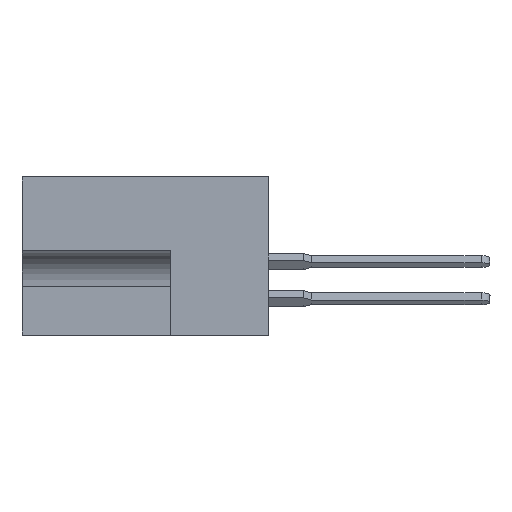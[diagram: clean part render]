
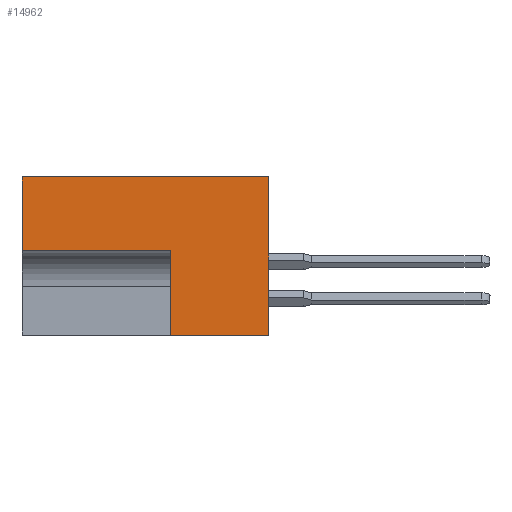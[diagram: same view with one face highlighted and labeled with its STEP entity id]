
A CAD part, left-side view. The second image highlights one B-rep face of the part: STEP entity #14962.
In plain terms, the highlighted planar face has unit normal (-1, 0, 0).
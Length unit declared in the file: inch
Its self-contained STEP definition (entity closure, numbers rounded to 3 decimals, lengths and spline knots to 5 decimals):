
#10 = DIRECTION ( 'NONE',  ( 0., 0., 1. ) ) ;
#1063 = LINE ( 'NONE', #12651, #9560 ) ;
#1127 = CARTESIAN_POINT ( 'NONE',  ( 0., 0.328, -0.248 ) ) ;
#2251 = DIRECTION ( 'NONE',  ( 0., -1., 0. ) ) ;
#2366 = VERTEX_POINT ( 'NONE', #2462 ) ;
#2462 = CARTESIAN_POINT ( 'NONE',  ( 0., 0., 0. ) ) ;
#3559 = DIRECTION ( 'NONE',  ( 0., 0., 1. ) ) ;
#3763 = ORIENTED_EDGE ( 'NONE', *, *, #11662, .F. ) ;
#5465 = VECTOR ( 'NONE', #10, 39.37008 ) ;
#5806 = ORIENTED_EDGE ( 'NONE', *, *, #26258, .T. ) ;
#5829 = VECTOR ( 'NONE', #8602, 39.37008 ) ;
#6051 = CARTESIAN_POINT ( 'NONE',  ( 0., 0.453, 0. ) ) ;
#6101 = ORIENTED_EDGE ( 'NONE', *, *, #23024, .T. ) ;
#6243 = VERTEX_POINT ( 'NONE', #10524 ) ;
#7580 = CARTESIAN_POINT ( 'NONE',  ( 0., 0.328, -0.531 ) ) ;
#8602 = DIRECTION ( 'NONE',  ( 0., 0., 1. ) ) ;
#9388 = EDGE_CURVE ( 'NONE', #23290, #2366, #15362, .T. ) ;
#9560 = VECTOR ( 'NONE', #2251, 39.37008 ) ;
#10290 = CARTESIAN_POINT ( 'NONE',  ( 0., 0., 0. ) ) ;
#10362 = LINE ( 'NONE', #10290, #5465 ) ;
#10475 = VECTOR ( 'NONE', #19140, 39.37008 ) ;
#10524 = CARTESIAN_POINT ( 'NONE',  ( 0., 0.328, -0.531 ) ) ;
#10763 = ORIENTED_EDGE ( 'NONE', *, *, #9388, .F. ) ;
#10971 = VERTEX_POINT ( 'NONE', #1127 ) ;
#11045 = LINE ( 'NONE', #16921, #5829 ) ;
#11230 = EDGE_CURVE ( 'NONE', #14862, #23290, #11045, .T. ) ;
#11662 = EDGE_CURVE ( 'NONE', #6243, #10971, #18782, .T. ) ;
#12002 = VECTOR ( 'NONE', #3559, 39.37008 ) ;
#12344 = DIRECTION ( 'NONE',  ( 0., -1., 0. ) ) ;
#12651 = CARTESIAN_POINT ( 'NONE',  ( 0., 0.453, -0.531 ) ) ;
#13093 = CARTESIAN_POINT ( 'NONE',  ( 0., 0.328, -0.248 ) ) ;
#13828 = PLANE ( 'NONE',  #17831 ) ;
#14303 = EDGE_LOOP ( 'NONE', ( #17032, #26651, #3763, #6101, #5806, #10763 ) ) ;
#14862 = VERTEX_POINT ( 'NONE', #25957 ) ;
#14962 = ADVANCED_FACE ( 'NONE', ( #21248 ), #13828, .F. ) ;
#15321 = LINE ( 'NONE', #13093, #10475 ) ;
#15362 = LINE ( 'NONE', #6051, #22157 ) ;
#15907 = CARTESIAN_POINT ( 'NONE',  ( 0., 0.453, 0. ) ) ;
#16921 = CARTESIAN_POINT ( 'NONE',  ( 0., 0.828, 0. ) ) ;
#17032 = ORIENTED_EDGE ( 'NONE', *, *, #11230, .F. ) ;
#17831 = AXIS2_PLACEMENT_3D ( 'NONE', #15907, #20251, #22413 ) ;
#18782 = LINE ( 'NONE', #7580, #12002 ) ;
#19140 = DIRECTION ( 'NONE',  ( 0., 1., 0. ) ) ;
#19229 = CARTESIAN_POINT ( 'NONE',  ( 0., 0., -0.531 ) ) ;
#19582 = CARTESIAN_POINT ( 'NONE',  ( 0., 0.828, 0. ) ) ;
#20251 = DIRECTION ( 'NONE',  ( 1., 0., 0. ) ) ;
#21248 = FACE_OUTER_BOUND ( 'NONE', #14303, .T. ) ;
#22157 = VECTOR ( 'NONE', #12344, 39.37008 ) ;
#22413 = DIRECTION ( 'NONE',  ( 0., 0., -1. ) ) ;
#23024 = EDGE_CURVE ( 'NONE', #6243, #23094, #1063, .T. ) ;
#23094 = VERTEX_POINT ( 'NONE', #19229 ) ;
#23290 = VERTEX_POINT ( 'NONE', #19582 ) ;
#24586 = EDGE_CURVE ( 'NONE', #10971, #14862, #15321, .T. ) ;
#25957 = CARTESIAN_POINT ( 'NONE',  ( 0., 0.828, -0.248 ) ) ;
#26258 = EDGE_CURVE ( 'NONE', #23094, #2366, #10362, .T. ) ;
#26651 = ORIENTED_EDGE ( 'NONE', *, *, #24586, .F. ) ;
